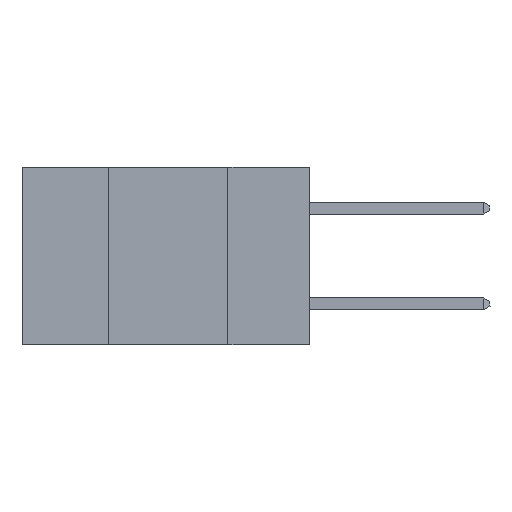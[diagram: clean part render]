
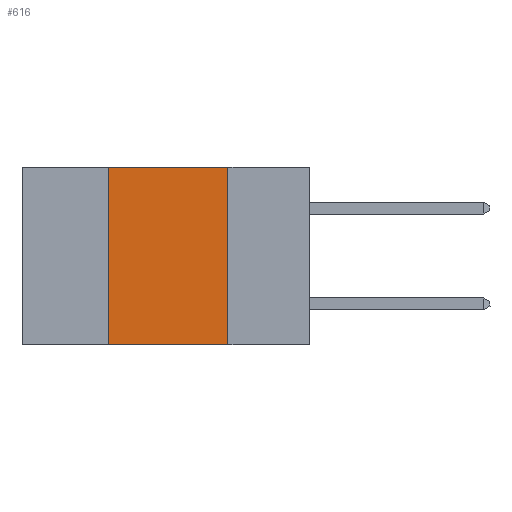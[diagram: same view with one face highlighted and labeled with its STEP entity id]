
A CAD part, left-side view. The second image highlights one B-rep face of the part: STEP entity #616.
In plain terms, the highlighted planar face has unit normal (-1, 0, 0).
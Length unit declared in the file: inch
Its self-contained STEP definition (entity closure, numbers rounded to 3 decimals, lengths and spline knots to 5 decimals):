
#347 = FACE_OUTER_BOUND ( 'NONE', #3682, .T. ) ;
#616 = ADVANCED_FACE ( 'NONE', ( #347 ), #4085, .F. ) ;
#999 = DIRECTION ( 'NONE',  ( 1., 0., 0. ) ) ;
#1246 = CARTESIAN_POINT ( 'NONE',  ( 0., 0.6, 0. ) ) ;
#1727 = VECTOR ( 'NONE', #11866, 39.37008 ) ;
#2251 = CARTESIAN_POINT ( 'NONE',  ( 0., 0.42, 0. ) ) ;
#2775 = VERTEX_POINT ( 'NONE', #2251 ) ;
#2909 = DIRECTION ( 'NONE',  ( 0., 0., -1. ) ) ;
#2942 = DIRECTION ( 'NONE',  ( 0., 0., -1. ) ) ;
#3018 = DIRECTION ( 'NONE',  ( 0., -1., 0. ) ) ;
#3037 = EDGE_CURVE ( 'NONE', #5710, #9715, #4814, .T. ) ;
#3351 = LINE ( 'NONE', #1246, #5001 ) ;
#3475 = ORIENTED_EDGE ( 'NONE', *, *, #10587, .F. ) ;
#3679 = ORIENTED_EDGE ( 'NONE', *, *, #7033, .F. ) ;
#3682 = EDGE_LOOP ( 'NONE', ( #3679, #5620, #3475, #8807 ) ) ;
#4085 = PLANE ( 'NONE',  #9442 ) ;
#4144 = VECTOR ( 'NONE', #2942, 39.37008 ) ;
#4814 = LINE ( 'NONE', #8865, #1727 ) ;
#5001 = VECTOR ( 'NONE', #3018, 39.37008 ) ;
#5620 = ORIENTED_EDGE ( 'NONE', *, *, #7964, .F. ) ;
#5710 = VERTEX_POINT ( 'NONE', #6998 ) ;
#6998 = CARTESIAN_POINT ( 'NONE',  ( 0., 0.42, -0.37 ) ) ;
#7033 = EDGE_CURVE ( 'NONE', #11969, #9715, #12184, .T. ) ;
#7111 = CARTESIAN_POINT ( 'NONE',  ( 0., 0.6, 0. ) ) ;
#7783 = CARTESIAN_POINT ( 'NONE',  ( 0., 0.17, 0. ) ) ;
#7964 = EDGE_CURVE ( 'NONE', #2775, #11969, #3351, .T. ) ;
#8724 = CARTESIAN_POINT ( 'NONE',  ( 0., 0.17, 0. ) ) ;
#8807 = ORIENTED_EDGE ( 'NONE', *, *, #3037, .T. ) ;
#8865 = CARTESIAN_POINT ( 'NONE',  ( 0., 0.6, -0.37 ) ) ;
#9442 = AXIS2_PLACEMENT_3D ( 'NONE', #7111, #999, #2909 ) ;
#9521 = DIRECTION ( 'NONE',  ( 0., 0., 1. ) ) ;
#9600 = VECTOR ( 'NONE', #9521, 39.37008 ) ;
#9715 = VERTEX_POINT ( 'NONE', #11119 ) ;
#10587 = EDGE_CURVE ( 'NONE', #5710, #2775, #12150, .T. ) ;
#11119 = CARTESIAN_POINT ( 'NONE',  ( 0., 0.17, -0.37 ) ) ;
#11487 = CARTESIAN_POINT ( 'NONE',  ( 0., 0.42, 0. ) ) ;
#11866 = DIRECTION ( 'NONE',  ( 0., -1., 0. ) ) ;
#11969 = VERTEX_POINT ( 'NONE', #7783 ) ;
#12150 = LINE ( 'NONE', #11487, #9600 ) ;
#12184 = LINE ( 'NONE', #8724, #4144 ) ;
